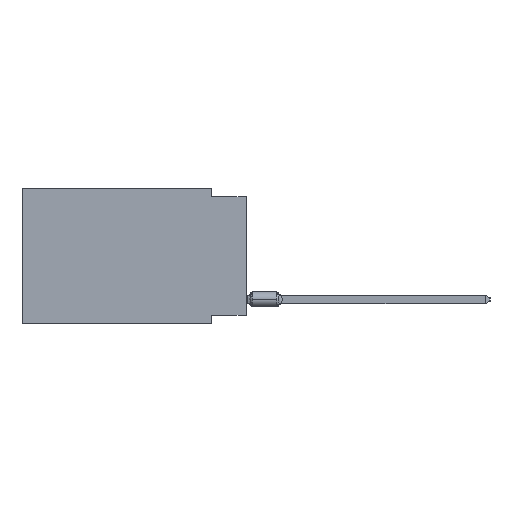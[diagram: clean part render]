
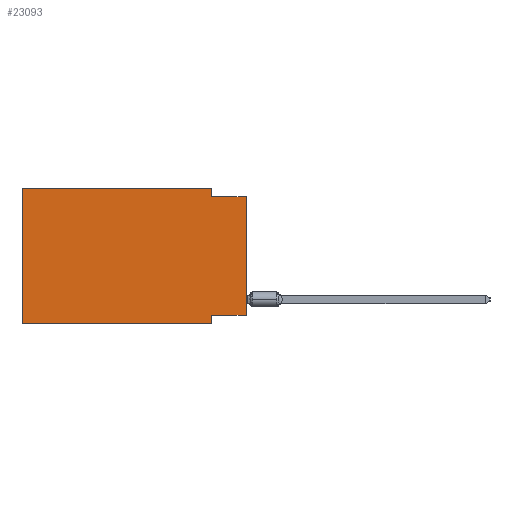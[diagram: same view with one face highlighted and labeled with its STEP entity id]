
A CAD part, left-side view. The second image highlights one B-rep face of the part: STEP entity #23093.
In plain terms, the highlighted planar face has unit normal (-1, 0, 0).
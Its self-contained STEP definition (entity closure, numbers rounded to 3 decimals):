
#900 = EDGE_CURVE ( 'NONE', #67808, #67402, #72086, .T. ) ;
#1261 = ORIENTED_EDGE ( 'NONE', *, *, #45752, .F. ) ;
#2172 = CARTESIAN_POINT ( 'NONE',  ( 0., 2.54, -9.271 ) ) ;
#3317 = LINE ( 'NONE', #51341, #7996 ) ;
#4134 = CARTESIAN_POINT ( 'NONE',  ( 0., 2.54, -9.906 ) ) ;
#5063 = DIRECTION ( 'NONE',  ( 1., 0., 0. ) ) ;
#5461 = CARTESIAN_POINT ( 'NONE',  ( 0., 16.383, 0. ) ) ;
#7996 = VECTOR ( 'NONE', #27133, 1000. ) ;
#8023 = CARTESIAN_POINT ( 'NONE',  ( 0., 16.383, 0. ) ) ;
#10078 = VERTEX_POINT ( 'NONE', #55309 ) ;
#11391 = CARTESIAN_POINT ( 'NONE',  ( 0., 2.54, 0. ) ) ;
#11515 = ORIENTED_EDGE ( 'NONE', *, *, #29037, .F. ) ;
#11844 = LINE ( 'NONE', #48339, #48785 ) ;
#15820 = VECTOR ( 'NONE', #18091, 1000. ) ;
#16216 = LINE ( 'NONE', #65422, #36637 ) ;
#17316 = CARTESIAN_POINT ( 'NONE',  ( 0., 0., 0. ) ) ;
#18091 = DIRECTION ( 'NONE',  ( 0., 0., 1. ) ) ;
#19596 = ORIENTED_EDGE ( 'NONE', *, *, #68503, .F. ) ;
#20398 = CARTESIAN_POINT ( 'NONE',  ( 0., 16.383, 0. ) ) ;
#21819 = VECTOR ( 'NONE', #36342, 1000. ) ;
#21931 = VECTOR ( 'NONE', #49761, 1000. ) ;
#23093 = ADVANCED_FACE ( 'NONE', ( #46759 ), #60225, .F. ) ;
#25399 = ORIENTED_EDGE ( 'NONE', *, *, #900, .T. ) ;
#25686 = CARTESIAN_POINT ( 'NONE',  ( 0., 0., -9.271 ) ) ;
#27133 = DIRECTION ( 'NONE',  ( 0., -1., 0. ) ) ;
#27917 = ORIENTED_EDGE ( 'NONE', *, *, #63652, .F. ) ;
#29037 = EDGE_CURVE ( 'NONE', #10078, #60782, #16216, .T. ) ;
#31245 = CARTESIAN_POINT ( 'NONE',  ( 0., 2.54, -9.906 ) ) ;
#32163 = AXIS2_PLACEMENT_3D ( 'NONE', #5461, #5063, #53888 ) ;
#32431 = DIRECTION ( 'NONE',  ( 0., 1., 0. ) ) ;
#32737 = EDGE_CURVE ( 'NONE', #60782, #53522, #49361, .T. ) ;
#32807 = LINE ( 'NONE', #25686, #72197 ) ;
#35263 = DIRECTION ( 'NONE',  ( 0., -1., 0. ) ) ;
#36342 = DIRECTION ( 'NONE',  ( 0., 0., -1. ) ) ;
#36637 = VECTOR ( 'NONE', #76172, 1000. ) ;
#39487 = ORIENTED_EDGE ( 'NONE', *, *, #60506, .F. ) ;
#45752 = EDGE_CURVE ( 'NONE', #68573, #67402, #11844, .T. ) ;
#46759 = FACE_OUTER_BOUND ( 'NONE', #49422, .T. ) ;
#46857 = VECTOR ( 'NONE', #76810, 1000. ) ;
#48245 = LINE ( 'NONE', #49029, #21819 ) ;
#48339 = CARTESIAN_POINT ( 'NONE',  ( 0., 0., -0.635 ) ) ;
#48785 = VECTOR ( 'NONE', #35263, 1000. ) ;
#49029 = CARTESIAN_POINT ( 'NONE',  ( 0., 2.54, 0. ) ) ;
#49361 = LINE ( 'NONE', #20398, #21931 ) ;
#49422 = EDGE_LOOP ( 'NONE', ( #25399, #1261, #27917, #74112, #11515, #53234, #39487, #19596 ) ) ;
#49761 = DIRECTION ( 'NONE',  ( 0., -1., 0. ) ) ;
#51341 = CARTESIAN_POINT ( 'NONE',  ( 0., 16.383, -9.906 ) ) ;
#53234 = ORIENTED_EDGE ( 'NONE', *, *, #74861, .T. ) ;
#53522 = VERTEX_POINT ( 'NONE', #11391 ) ;
#53888 = DIRECTION ( 'NONE',  ( 0., 0., -1. ) ) ;
#55309 = CARTESIAN_POINT ( 'NONE',  ( 0., 16.383, -9.906 ) ) ;
#57933 = VERTEX_POINT ( 'NONE', #2172 ) ;
#58509 = LINE ( 'NONE', #4134, #46857 ) ;
#58779 = CARTESIAN_POINT ( 'NONE',  ( 0., 0., -9.271 ) ) ;
#60225 = PLANE ( 'NONE',  #32163 ) ;
#60506 = EDGE_CURVE ( 'NONE', #57933, #68339, #58509, .T. ) ;
#60782 = VERTEX_POINT ( 'NONE', #8023 ) ;
#63652 = EDGE_CURVE ( 'NONE', #53522, #68573, #48245, .T. ) ;
#65343 = CARTESIAN_POINT ( 'NONE',  ( 0., 0., -0.635 ) ) ;
#65354 = CARTESIAN_POINT ( 'NONE',  ( 0., 2.54, -0.635 ) ) ;
#65422 = CARTESIAN_POINT ( 'NONE',  ( 0., 16.383, 0. ) ) ;
#67402 = VERTEX_POINT ( 'NONE', #65343 ) ;
#67808 = VERTEX_POINT ( 'NONE', #58779 ) ;
#68339 = VERTEX_POINT ( 'NONE', #31245 ) ;
#68503 = EDGE_CURVE ( 'NONE', #67808, #57933, #32807, .T. ) ;
#68573 = VERTEX_POINT ( 'NONE', #65354 ) ;
#72086 = LINE ( 'NONE', #17316, #15820 ) ;
#72197 = VECTOR ( 'NONE', #32431, 1000. ) ;
#74112 = ORIENTED_EDGE ( 'NONE', *, *, #32737, .F. ) ;
#74861 = EDGE_CURVE ( 'NONE', #10078, #68339, #3317, .T. ) ;
#76172 = DIRECTION ( 'NONE',  ( 0., 0., 1. ) ) ;
#76810 = DIRECTION ( 'NONE',  ( 0., 0., -1. ) ) ;
